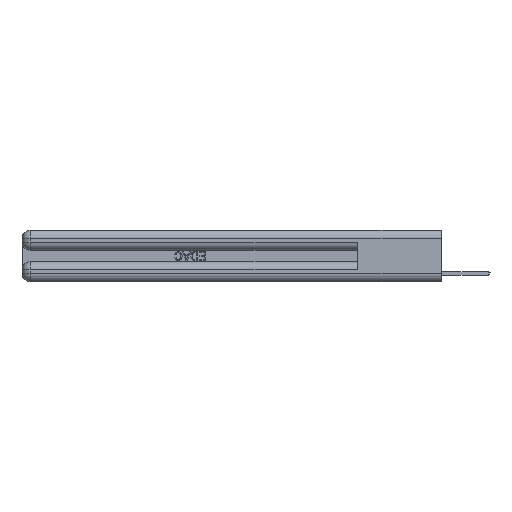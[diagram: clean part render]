
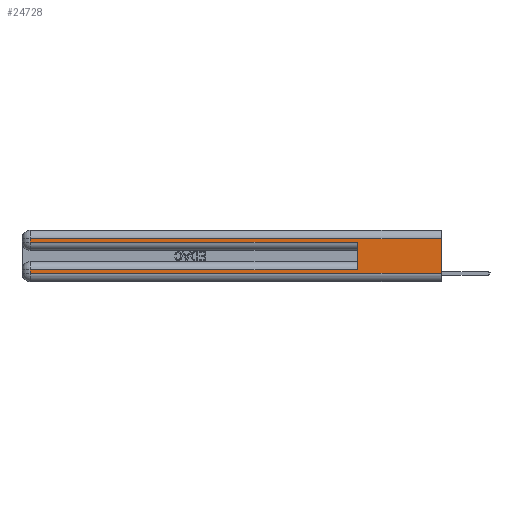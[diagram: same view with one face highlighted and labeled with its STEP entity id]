
A CAD part, left-side view. The second image highlights one B-rep face of the part: STEP entity #24728.
In plain terms, the highlighted planar face has unit normal (-1, 0, 0).
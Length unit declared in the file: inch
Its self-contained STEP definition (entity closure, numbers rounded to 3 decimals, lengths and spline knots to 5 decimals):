
#148 = CARTESIAN_POINT ( 'NONE',  ( 0., 2.94, 0.31 ) ) ;
#193 = LINE ( 'NONE', #26860, #19978 ) ;
#249 = ORIENTED_EDGE ( 'NONE', *, *, #14799, .F. ) ;
#373 = ORIENTED_EDGE ( 'NONE', *, *, #23728, .F. ) ;
#1085 = DIRECTION ( 'NONE',  ( 0., 0., -1. ) ) ;
#1597 = VERTEX_POINT ( 'NONE', #18701 ) ;
#1977 = FACE_OUTER_BOUND ( 'NONE', #4155, .T. ) ;
#3390 = LINE ( 'NONE', #5597, #20392 ) ;
#3540 = LINE ( 'NONE', #8440, #17471 ) ;
#3700 = ORIENTED_EDGE ( 'NONE', *, *, #17343, .T. ) ;
#4155 = EDGE_LOOP ( 'NONE', ( #249, #3700, #8724, #21050, #373, #12670, #28265, #7253 ) ) ;
#4771 = AXIS2_PLACEMENT_3D ( 'NONE', #11050, #27617, #17827 ) ;
#5597 = CARTESIAN_POINT ( 'NONE',  ( 0., 0.6, 0.145 ) ) ;
#6204 = CARTESIAN_POINT ( 'NONE',  ( 0., 0., 0.06 ) ) ;
#7187 = VERTEX_POINT ( 'NONE', #15838 ) ;
#7253 = ORIENTED_EDGE ( 'NONE', *, *, #31209, .T. ) ;
#7274 = VERTEX_POINT ( 'NONE', #30834 ) ;
#7481 = EDGE_CURVE ( 'NONE', #14122, #1597, #193, .T. ) ;
#7860 = VECTOR ( 'NONE', #14183, 39.37008 ) ;
#8129 = DIRECTION ( 'NONE',  ( 0., -1., 0. ) ) ;
#8203 = PLANE ( 'NONE',  #4771 ) ;
#8440 = CARTESIAN_POINT ( 'NONE',  ( 0., 0., 0.285 ) ) ;
#8724 = ORIENTED_EDGE ( 'NONE', *, *, #15852, .T. ) ;
#8825 = CARTESIAN_POINT ( 'NONE',  ( 0., 0., 0.37 ) ) ;
#9178 = VERTEX_POINT ( 'NONE', #25103 ) ;
#10256 = LINE ( 'NONE', #12940, #23657 ) ;
#11050 = CARTESIAN_POINT ( 'NONE',  ( 0., 0., 0.37 ) ) ;
#12670 = ORIENTED_EDGE ( 'NONE', *, *, #7481, .T. ) ;
#12940 = CARTESIAN_POINT ( 'NONE',  ( 0., 2.94, 0.37 ) ) ;
#13260 = CARTESIAN_POINT ( 'NONE',  ( 0., 0., 0.31 ) ) ;
#14122 = VERTEX_POINT ( 'NONE', #26270 ) ;
#14183 = DIRECTION ( 'NONE',  ( 0., 0., -1. ) ) ;
#14412 = DIRECTION ( 'NONE',  ( 0., 1., 0. ) ) ;
#14799 = EDGE_CURVE ( 'NONE', #15105, #18894, #25549, .T. ) ;
#15105 = VERTEX_POINT ( 'NONE', #20471 ) ;
#15632 = DIRECTION ( 'NONE',  ( 0., 1., 0. ) ) ;
#15838 = CARTESIAN_POINT ( 'NONE',  ( 0., 2.94, 0.285 ) ) ;
#15852 = EDGE_CURVE ( 'NONE', #28929, #7187, #17856, .T. ) ;
#17343 = EDGE_CURVE ( 'NONE', #15105, #28929, #23029, .T. ) ;
#17471 = VECTOR ( 'NONE', #8129, 39.37008 ) ;
#17827 = DIRECTION ( 'NONE',  ( 0., 0., -1. ) ) ;
#17856 = LINE ( 'NONE', #25266, #21970 ) ;
#18300 = EDGE_CURVE ( 'NONE', #7187, #7274, #3540, .T. ) ;
#18701 = CARTESIAN_POINT ( 'NONE',  ( 0., 2.94, 0.085 ) ) ;
#18894 = VERTEX_POINT ( 'NONE', #23833 ) ;
#19978 = VECTOR ( 'NONE', #14412, 39.37008 ) ;
#20392 = VECTOR ( 'NONE', #29912, 39.37008 ) ;
#20471 = CARTESIAN_POINT ( 'NONE',  ( 0., 0., 0.31 ) ) ;
#20871 = LINE ( 'NONE', #6204, #29742 ) ;
#21050 = ORIENTED_EDGE ( 'NONE', *, *, #18300, .T. ) ;
#21966 = VECTOR ( 'NONE', #15632, 39.37008 ) ;
#21970 = VECTOR ( 'NONE', #23067, 39.37008 ) ;
#23029 = LINE ( 'NONE', #13260, #21966 ) ;
#23067 = DIRECTION ( 'NONE',  ( 0., 0., -1. ) ) ;
#23552 = DIRECTION ( 'NONE',  ( 0., -1., 0. ) ) ;
#23657 = VECTOR ( 'NONE', #1085, 39.37008 ) ;
#23728 = EDGE_CURVE ( 'NONE', #14122, #7274, #3390, .T. ) ;
#23833 = CARTESIAN_POINT ( 'NONE',  ( 0., 0., 0.06 ) ) ;
#24728 = ADVANCED_FACE ( 'NONE', ( #1977 ), #8203, .F. ) ;
#25103 = CARTESIAN_POINT ( 'NONE',  ( 0., 2.94, 0.06 ) ) ;
#25266 = CARTESIAN_POINT ( 'NONE',  ( 0., 2.94, 0.37 ) ) ;
#25549 = LINE ( 'NONE', #8825, #7860 ) ;
#26270 = CARTESIAN_POINT ( 'NONE',  ( 0., 0.6, 0.085 ) ) ;
#26860 = CARTESIAN_POINT ( 'NONE',  ( 0., 0., 0.085 ) ) ;
#27617 = DIRECTION ( 'NONE',  ( 1., 0., 0. ) ) ;
#28265 = ORIENTED_EDGE ( 'NONE', *, *, #29035, .T. ) ;
#28929 = VERTEX_POINT ( 'NONE', #148 ) ;
#29035 = EDGE_CURVE ( 'NONE', #1597, #9178, #10256, .T. ) ;
#29742 = VECTOR ( 'NONE', #23552, 39.37008 ) ;
#29912 = DIRECTION ( 'NONE',  ( 0., 0., 1. ) ) ;
#30834 = CARTESIAN_POINT ( 'NONE',  ( 0., 0.6, 0.285 ) ) ;
#31209 = EDGE_CURVE ( 'NONE', #9178, #18894, #20871, .T. ) ;
